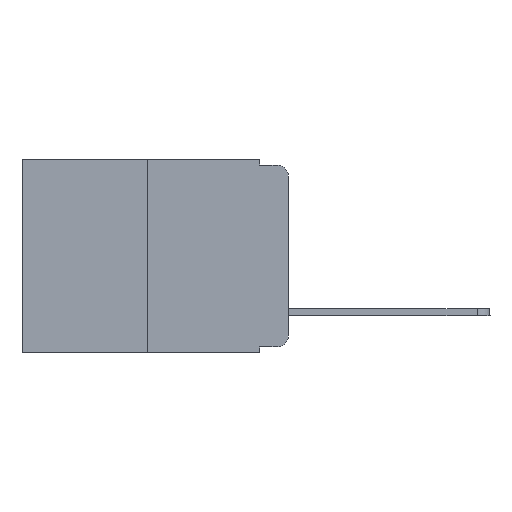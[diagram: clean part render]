
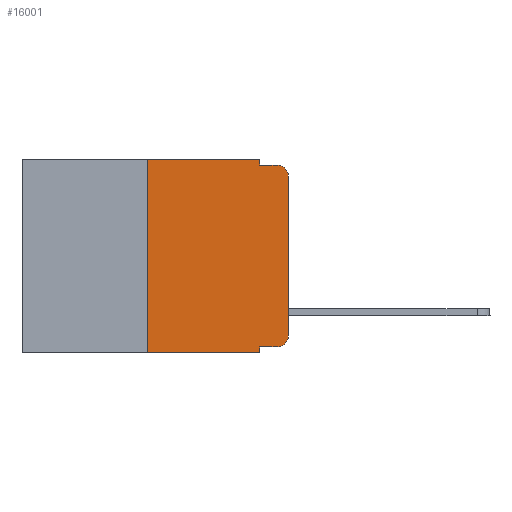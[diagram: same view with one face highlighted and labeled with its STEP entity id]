
A CAD part, left-side view. The second image highlights one B-rep face of the part: STEP entity #16001.
In plain terms, the highlighted planar face has unit normal (-1, 0, 0).
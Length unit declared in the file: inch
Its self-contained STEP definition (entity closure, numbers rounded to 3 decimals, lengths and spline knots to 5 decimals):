
#223 = EDGE_CURVE ( 'NONE', #3101, #9799, #20086, .T. ) ;
#454 = AXIS2_PLACEMENT_3D ( 'NONE', #21780, #2734, #14878 ) ;
#565 = AXIS2_PLACEMENT_3D ( 'NONE', #4229, #9188, #3999 ) ;
#932 = DIRECTION ( 'NONE',  ( 0., -1., 0. ) ) ;
#948 = EDGE_CURVE ( 'NONE', #7948, #5894, #7873, .T. ) ;
#1395 = LINE ( 'NONE', #11242, #12503 ) ;
#2061 = DIRECTION ( 'NONE',  ( 0., 0., -1. ) ) ;
#2579 = DIRECTION ( 'NONE',  ( 0., 0., 1. ) ) ;
#2709 = VERTEX_POINT ( 'NONE', #17530 ) ;
#2734 = DIRECTION ( 'NONE',  ( 1., 0., 0. ) ) ;
#2777 = LINE ( 'NONE', #8747, #21790 ) ;
#3101 = VERTEX_POINT ( 'NONE', #14108 ) ;
#3309 = EDGE_CURVE ( 'NONE', #2709, #7948, #17788, .T. ) ;
#3474 = CARTESIAN_POINT ( 'NONE',  ( 0., 0.051, -0.01 ) ) ;
#3706 = CARTESIAN_POINT ( 'NONE',  ( 0., 0., -0.313 ) ) ;
#3999 = DIRECTION ( 'NONE',  ( 0., 0., -1. ) ) ;
#4101 = DIRECTION ( 'NONE',  ( 0., 0., -1. ) ) ;
#4229 = CARTESIAN_POINT ( 'NONE',  ( 0., 0.02, -0.313 ) ) ;
#4882 = VECTOR ( 'NONE', #21542, 39.37008 ) ;
#5304 = EDGE_CURVE ( 'NONE', #20356, #2709, #21551, .T. ) ;
#5543 = LINE ( 'NONE', #19945, #14236 ) ;
#5894 = VERTEX_POINT ( 'NONE', #13272 ) ;
#6040 = EDGE_CURVE ( 'NONE', #9799, #22179, #1395, .T. ) ;
#6041 = VERTEX_POINT ( 'NONE', #13060 ) ;
#6294 = ORIENTED_EDGE ( 'NONE', *, *, #948, .T. ) ;
#6527 = VECTOR ( 'NONE', #2061, 39.37008 ) ;
#6871 = AXIS2_PLACEMENT_3D ( 'NONE', #10800, #14445, #4101 ) ;
#7361 = VERTEX_POINT ( 'NONE', #21669 ) ;
#7873 = LINE ( 'NONE', #19841, #4882 ) ;
#7948 = VERTEX_POINT ( 'NONE', #3706 ) ;
#8136 = ORIENTED_EDGE ( 'NONE', *, *, #14060, .F. ) ;
#8747 = CARTESIAN_POINT ( 'NONE',  ( 0., 0.473, 0. ) ) ;
#8769 = ORIENTED_EDGE ( 'NONE', *, *, #21274, .F. ) ;
#8950 = ORIENTED_EDGE ( 'NONE', *, *, #3309, .T. ) ;
#9188 = DIRECTION ( 'NONE',  ( -1., 0., 0. ) ) ;
#9691 = EDGE_CURVE ( 'NONE', #16823, #7361, #5543, .T. ) ;
#9799 = VERTEX_POINT ( 'NONE', #3474 ) ;
#10800 = CARTESIAN_POINT ( 'NONE',  ( 0., 0.02, -0.03 ) ) ;
#11242 = CARTESIAN_POINT ( 'NONE',  ( 0., 0.051, -0.01 ) ) ;
#12327 = DIRECTION ( 'NONE',  ( 0., 0., -1. ) ) ;
#12485 = FACE_OUTER_BOUND ( 'NONE', #13288, .T. ) ;
#12503 = VECTOR ( 'NONE', #932, 39.37008 ) ;
#13060 = CARTESIAN_POINT ( 'NONE',  ( 0., 0.25, 0. ) ) ;
#13272 = CARTESIAN_POINT ( 'NONE',  ( 0., 0., -0.03 ) ) ;
#13288 = EDGE_LOOP ( 'NONE', ( #6294, #14507, #20407, #14592, #13379, #8136, #21543, #8769, #21022, #8950 ) ) ;
#13379 = ORIENTED_EDGE ( 'NONE', *, *, #19551, .F. ) ;
#13623 = VECTOR ( 'NONE', #2579, 39.37008 ) ;
#14060 = EDGE_CURVE ( 'NONE', #16823, #6041, #17140, .T. ) ;
#14108 = CARTESIAN_POINT ( 'NONE',  ( 0., 0.051, 0. ) ) ;
#14236 = VECTOR ( 'NONE', #19859, 39.37008 ) ;
#14445 = DIRECTION ( 'NONE',  ( -1., 0., 0. ) ) ;
#14507 = ORIENTED_EDGE ( 'NONE', *, *, #16742, .T. ) ;
#14592 = ORIENTED_EDGE ( 'NONE', *, *, #223, .F. ) ;
#14878 = DIRECTION ( 'NONE',  ( 0., 0., -1. ) ) ;
#14946 = CARTESIAN_POINT ( 'NONE',  ( 0., 0.02, -0.01 ) ) ;
#15057 = DIRECTION ( 'NONE',  ( 0., -1., 0. ) ) ;
#15656 = DIRECTION ( 'NONE',  ( 0., -1., 0. ) ) ;
#16001 = ADVANCED_FACE ( 'NONE', ( #12485 ), #16534, .F. ) ;
#16237 = CIRCLE ( 'NONE', #6871, 0.02 ) ;
#16534 = PLANE ( 'NONE',  #454 ) ;
#16742 = EDGE_CURVE ( 'NONE', #5894, #22179, #16237, .T. ) ;
#16823 = VERTEX_POINT ( 'NONE', #19342 ) ;
#16907 = VECTOR ( 'NONE', #15057, 39.37008 ) ;
#17140 = LINE ( 'NONE', #21778, #13623 ) ;
#17160 = CARTESIAN_POINT ( 'NONE',  ( 0., 0.051, 0. ) ) ;
#17530 = CARTESIAN_POINT ( 'NONE',  ( 0., 0.02, -0.333 ) ) ;
#17619 = LINE ( 'NONE', #17160, #22249 ) ;
#17788 = CIRCLE ( 'NONE', #565, 0.02 ) ;
#19342 = CARTESIAN_POINT ( 'NONE',  ( 0., 0.25, -0.343 ) ) ;
#19551 = EDGE_CURVE ( 'NONE', #6041, #3101, #2777, .T. ) ;
#19841 = CARTESIAN_POINT ( 'NONE',  ( 0., 0., 0. ) ) ;
#19859 = DIRECTION ( 'NONE',  ( 0., -1., 0. ) ) ;
#19945 = CARTESIAN_POINT ( 'NONE',  ( 0., 0.473, -0.343 ) ) ;
#20086 = LINE ( 'NONE', #21322, #6527 ) ;
#20356 = VERTEX_POINT ( 'NONE', #21688 ) ;
#20407 = ORIENTED_EDGE ( 'NONE', *, *, #6040, .F. ) ;
#21022 = ORIENTED_EDGE ( 'NONE', *, *, #5304, .T. ) ;
#21274 = EDGE_CURVE ( 'NONE', #20356, #7361, #17619, .T. ) ;
#21322 = CARTESIAN_POINT ( 'NONE',  ( 0., 0.051, 0. ) ) ;
#21542 = DIRECTION ( 'NONE',  ( 0., 0., 1. ) ) ;
#21543 = ORIENTED_EDGE ( 'NONE', *, *, #9691, .T. ) ;
#21551 = LINE ( 'NONE', #22421, #16907 ) ;
#21669 = CARTESIAN_POINT ( 'NONE',  ( 0., 0.051, -0.343 ) ) ;
#21688 = CARTESIAN_POINT ( 'NONE',  ( 0., 0.051, -0.333 ) ) ;
#21778 = CARTESIAN_POINT ( 'NONE',  ( 0., 0.25, 0. ) ) ;
#21780 = CARTESIAN_POINT ( 'NONE',  ( 0., 0.473, 0. ) ) ;
#21790 = VECTOR ( 'NONE', #15656, 39.37008 ) ;
#22179 = VERTEX_POINT ( 'NONE', #14946 ) ;
#22249 = VECTOR ( 'NONE', #12327, 39.37008 ) ;
#22421 = CARTESIAN_POINT ( 'NONE',  ( 0., 0.051, -0.333 ) ) ;
